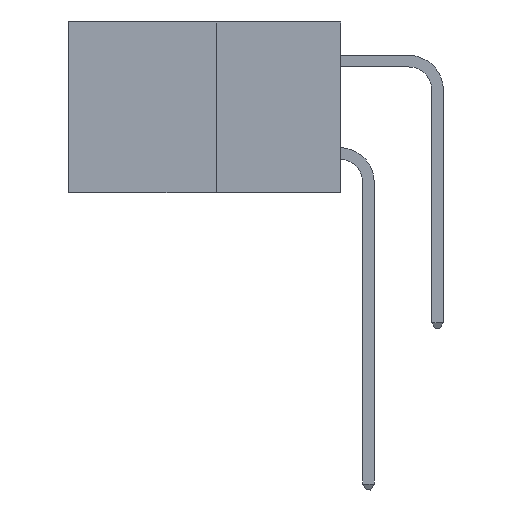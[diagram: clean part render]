
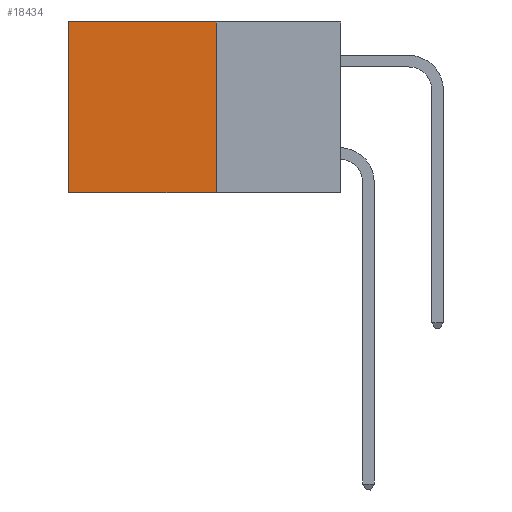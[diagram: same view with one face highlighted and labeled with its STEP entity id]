
A CAD part, left-side view. The second image highlights one B-rep face of the part: STEP entity #18434.
In plain terms, the highlighted planar face has unit normal (-1, 0, 0).
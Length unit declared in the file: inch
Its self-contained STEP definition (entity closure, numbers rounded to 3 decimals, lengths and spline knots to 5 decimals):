
#290 = CARTESIAN_POINT ( 'NONE',  ( 0.277, 0.27, -0.37 ) ) ;
#1475 = VECTOR ( 'NONE', #25243, 39.37008 ) ;
#1806 = VECTOR ( 'NONE', #20084, 39.37008 ) ;
#2426 = ORIENTED_EDGE ( 'NONE', *, *, #20043, .T. ) ;
#2892 = DIRECTION ( 'NONE',  ( 1., 0., 0. ) ) ;
#3657 = EDGE_CURVE ( 'NONE', #19651, #7470, #24753, .T. ) ;
#3958 = CARTESIAN_POINT ( 'NONE',  ( 0.277, 0.27, -0.37 ) ) ;
#4938 = EDGE_CURVE ( 'NONE', #29575, #29650, #15485, .T. ) ;
#5407 = DIRECTION ( 'NONE',  ( 0., 1., 0. ) ) ;
#7017 = VECTOR ( 'NONE', #17885, 39.37008 ) ;
#7470 = VERTEX_POINT ( 'NONE', #17100 ) ;
#7790 = PLANE ( 'NONE',  #8103 ) ;
#7911 = ORIENTED_EDGE ( 'NONE', *, *, #3657, .F. ) ;
#8047 = ORIENTED_EDGE ( 'NONE', *, *, #4938, .T. ) ;
#8103 = AXIS2_PLACEMENT_3D ( 'NONE', #15305, #2892, #20198 ) ;
#9945 = EDGE_LOOP ( 'NONE', ( #2426, #7911, #27679, #8047 ) ) ;
#12276 = CARTESIAN_POINT ( 'NONE',  ( 0.277, 0.59, 0. ) ) ;
#14486 = FACE_OUTER_BOUND ( 'NONE', #9945, .T. ) ;
#15305 = CARTESIAN_POINT ( 'NONE',  ( 0.277, 0.27, -0.37 ) ) ;
#15485 = LINE ( 'NONE', #25393, #1475 ) ;
#17100 = CARTESIAN_POINT ( 'NONE',  ( 0.277, 0.59, -0.37 ) ) ;
#17885 = DIRECTION ( 'NONE',  ( 0., 0., -1. ) ) ;
#18434 = ADVANCED_FACE ( 'NONE', ( #14486 ), #7790, .F. ) ;
#18870 = CARTESIAN_POINT ( 'NONE',  ( 0.277, 0.27, -0.37 ) ) ;
#19651 = VERTEX_POINT ( 'NONE', #18870 ) ;
#20043 = EDGE_CURVE ( 'NONE', #29650, #7470, #21712, .T. ) ;
#20084 = DIRECTION ( 'NONE',  ( 0., 0., -1. ) ) ;
#20198 = DIRECTION ( 'NONE',  ( 0., 0., -1. ) ) ;
#21524 = LINE ( 'NONE', #290, #1806 ) ;
#21712 = LINE ( 'NONE', #30096, #7017 ) ;
#22602 = EDGE_CURVE ( 'NONE', #29575, #19651, #21524, .T. ) ;
#24753 = LINE ( 'NONE', #3958, #30485 ) ;
#25243 = DIRECTION ( 'NONE',  ( 0., 1., 0. ) ) ;
#25393 = CARTESIAN_POINT ( 'NONE',  ( 0.277, 0.27, 0. ) ) ;
#26676 = CARTESIAN_POINT ( 'NONE',  ( 0.277, 0.27, 0. ) ) ;
#27679 = ORIENTED_EDGE ( 'NONE', *, *, #22602, .F. ) ;
#29575 = VERTEX_POINT ( 'NONE', #26676 ) ;
#29650 = VERTEX_POINT ( 'NONE', #12276 ) ;
#30096 = CARTESIAN_POINT ( 'NONE',  ( 0.277, 0.59, -0.37 ) ) ;
#30485 = VECTOR ( 'NONE', #5407, 39.37008 ) ;
